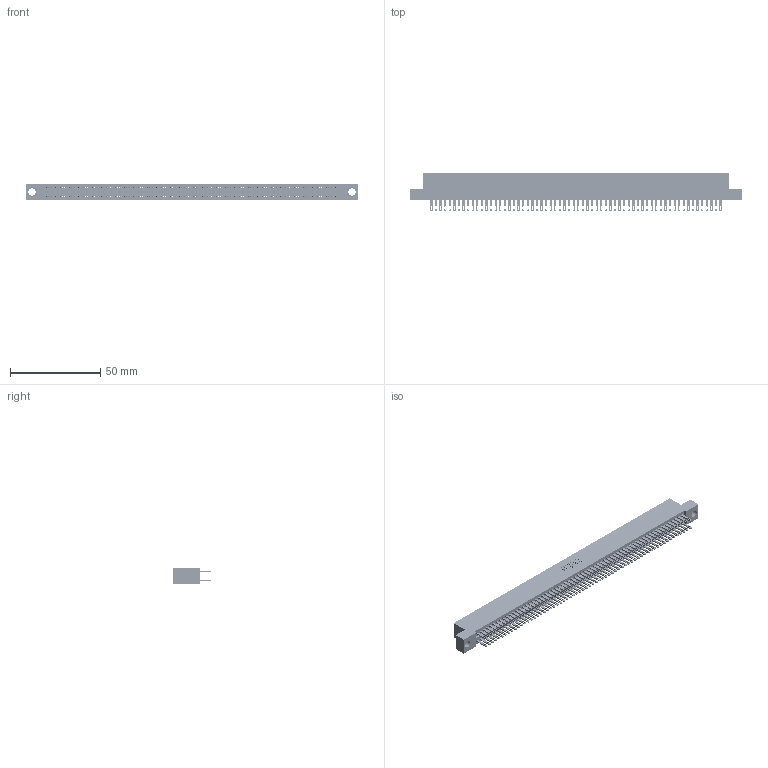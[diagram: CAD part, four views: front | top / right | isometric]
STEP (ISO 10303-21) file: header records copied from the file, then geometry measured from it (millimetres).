
FILE_DESCRIPTION (( 'STEP AP203' ), '1' );
FILE_NAME ('895-128-500-204.STEP', '2020-10-13T16:30:31', ( '' ), ( '' ), 'SwSTEP 2.0', 'SolidWorks 2020', '' );
FILE_SCHEMA (( 'CONFIG_CONTROL_DESIGN' ));
Length unit declared in the file: inch
Products named in the file (3): 345-292-001_345-293-100; 895-128-500-204; 845 Part_Flush Mounting Lugs - 0.156 Dia-TH
Assembly tree (129 placements, depth 2):
  895-128-500-204
    845 Part_Flush Mounting Lugs - 0.156 Dia-TH
    345-292-001_345-293-100  x128
Bounding box: 183.77 x 21.51 x 9.4 mm (x, y, z)
Volume: 18359 mm3; surface area: 28684.5 mm2
Topology: 129 solids, 129 shells, 6014 faces, 18389 edges, 12258 vertices
Faces by surface type: plane 3536, cylinder 2478
Entity records: 47187 total; most frequent: CARTESIAN_POINT 7888, ORIENTED_EDGE 7822, DIRECTION 6931, EDGE_CURVE 3911, VECTOR 3519, LINE 3519, VERTEX_POINT 2606, AXIS2_PLACEMENT_3D 1706
